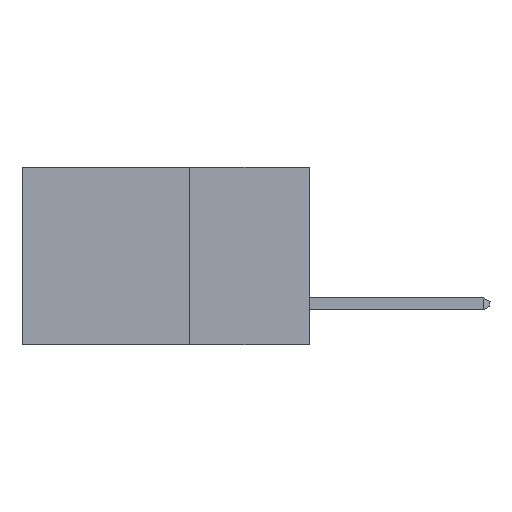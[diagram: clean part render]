
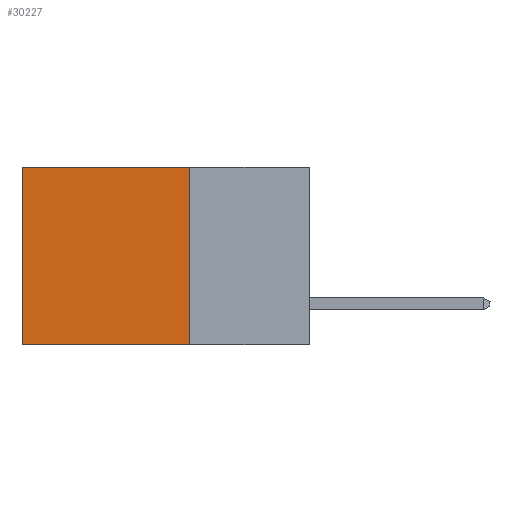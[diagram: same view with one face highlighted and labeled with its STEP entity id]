
A CAD part, left-side view. The second image highlights one B-rep face of the part: STEP entity #30227.
In plain terms, the highlighted planar face has unit normal (-1, 0, 0).
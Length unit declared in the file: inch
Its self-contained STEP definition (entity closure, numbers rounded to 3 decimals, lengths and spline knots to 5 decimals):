
#1456 = DIRECTION ( 'NONE',  ( 0., 0., -1. ) ) ;
#1879 = CARTESIAN_POINT ( 'NONE',  ( 0.2875, 0.25, -0.37 ) ) ;
#2025 = EDGE_CURVE ( 'NONE', #34047, #6070, #17163, .T. ) ;
#2811 = EDGE_CURVE ( 'NONE', #17463, #13468, #24535, .T. ) ;
#4027 = LINE ( 'NONE', #6688, #28184 ) ;
#4293 = CARTESIAN_POINT ( 'NONE',  ( 0.2875, 0.25, 0. ) ) ;
#5230 = ORIENTED_EDGE ( 'NONE', *, *, #2811, .F. ) ;
#5388 = DIRECTION ( 'NONE',  ( 0., 1., 0. ) ) ;
#6070 = VERTEX_POINT ( 'NONE', #36221 ) ;
#6688 = CARTESIAN_POINT ( 'NONE',  ( 0.2875, 0.25, 0. ) ) ;
#7501 = ORIENTED_EDGE ( 'NONE', *, *, #11688, .F. ) ;
#9923 = DIRECTION ( 'NONE',  ( 0., 0., -1. ) ) ;
#10060 = VECTOR ( 'NONE', #5388, 39.37008 ) ;
#10880 = ORIENTED_EDGE ( 'NONE', *, *, #18490, .T. ) ;
#11688 = EDGE_CURVE ( 'NONE', #34047, #17463, #4027, .T. ) ;
#12417 = VECTOR ( 'NONE', #12735, 39.37008 ) ;
#12735 = DIRECTION ( 'NONE',  ( 0., 1., 0. ) ) ;
#13468 = VERTEX_POINT ( 'NONE', #22651 ) ;
#15885 = DIRECTION ( 'NONE',  ( 1., 0., 0. ) ) ;
#17163 = LINE ( 'NONE', #34322, #10060 ) ;
#17463 = VERTEX_POINT ( 'NONE', #1879 ) ;
#18360 = CARTESIAN_POINT ( 'NONE',  ( 0.2875, 0.25, 0. ) ) ;
#18490 = EDGE_CURVE ( 'NONE', #6070, #13468, #20552, .T. ) ;
#19656 = AXIS2_PLACEMENT_3D ( 'NONE', #4293, #15885, #1456 ) ;
#20552 = LINE ( 'NONE', #21301, #34189 ) ;
#21301 = CARTESIAN_POINT ( 'NONE',  ( 0.2875, 0.6, 0. ) ) ;
#22651 = CARTESIAN_POINT ( 'NONE',  ( 0.2875, 0.6, -0.37 ) ) ;
#24470 = EDGE_LOOP ( 'NONE', ( #10880, #5230, #7501, #31211 ) ) ;
#24535 = LINE ( 'NONE', #24908, #12417 ) ;
#24908 = CARTESIAN_POINT ( 'NONE',  ( 0.2875, 0.25, -0.37 ) ) ;
#26820 = DIRECTION ( 'NONE',  ( 0., 0., -1. ) ) ;
#28184 = VECTOR ( 'NONE', #9923, 39.37008 ) ;
#30227 = ADVANCED_FACE ( 'NONE', ( #32690 ), #32500, .F. ) ;
#31211 = ORIENTED_EDGE ( 'NONE', *, *, #2025, .T. ) ;
#32500 = PLANE ( 'NONE',  #19656 ) ;
#32690 = FACE_OUTER_BOUND ( 'NONE', #24470, .T. ) ;
#34047 = VERTEX_POINT ( 'NONE', #18360 ) ;
#34189 = VECTOR ( 'NONE', #26820, 39.37008 ) ;
#34322 = CARTESIAN_POINT ( 'NONE',  ( 0.2875, 0.25, 0. ) ) ;
#36221 = CARTESIAN_POINT ( 'NONE',  ( 0.2875, 0.6, 0. ) ) ;
